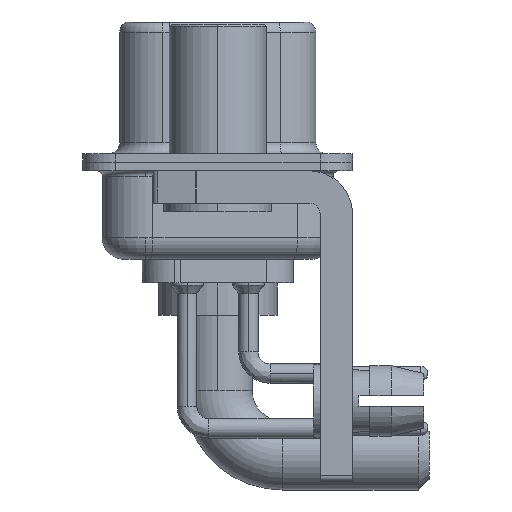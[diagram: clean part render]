
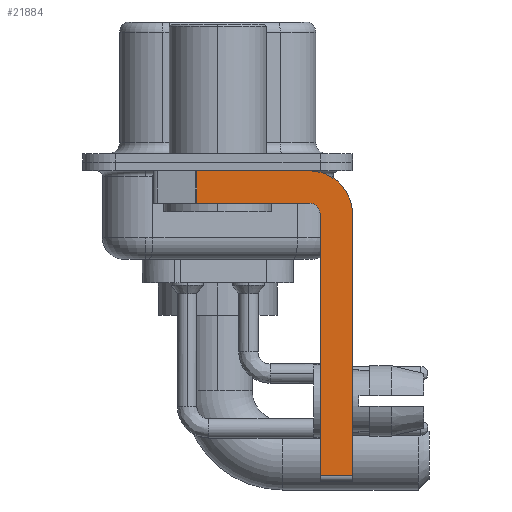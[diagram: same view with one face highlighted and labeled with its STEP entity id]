
A CAD part, left-side view. The second image highlights one B-rep face of the part: STEP entity #21884.
In plain terms, the highlighted planar face has unit normal (-1, 0, 0).
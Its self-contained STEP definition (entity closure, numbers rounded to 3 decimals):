
#239 = CARTESIAN_POINT ( 'NONE',  ( -2.9, 3., -0.4 ) ) ;
#353 = VERTEX_POINT ( 'NONE', #10017 ) ;
#521 = VERTEX_POINT ( 'NONE', #20869 ) ;
#617 = EDGE_CURVE ( 'NONE', #521, #15076, #24354, .T. ) ;
#702 = VECTOR ( 'NONE', #2770, 1000. ) ;
#852 = LINE ( 'NONE', #6659, #13976 ) ;
#1136 = DIRECTION ( 'NONE',  ( 0., 0., 1. ) ) ;
#1795 = DIRECTION ( 'NONE',  ( 0., 0., -1. ) ) ;
#1837 = EDGE_LOOP ( 'NONE', ( #18274, #26027, #17618, #20742, #22426, #16572, #10650, #2197 ) ) ;
#2197 = ORIENTED_EDGE ( 'NONE', *, *, #8988, .F. ) ;
#2770 = DIRECTION ( 'NONE',  ( 0., 1., 0. ) ) ;
#2832 = CARTESIAN_POINT ( 'NONE',  ( -2.9, -4.25, -0.4 ) ) ;
#2999 = DIRECTION ( 'NONE',  ( 0., -1., 0. ) ) ;
#4665 = LINE ( 'NONE', #6548, #12207 ) ;
#4983 = VERTEX_POINT ( 'NONE', #22659 ) ;
#5215 = DIRECTION ( 'NONE',  ( 0., 0., -1. ) ) ;
#5569 = AXIS2_PLACEMENT_3D ( 'NONE', #19363, #12936, #1136 ) ;
#5831 = VECTOR ( 'NONE', #2999, 1000. ) ;
#6110 = CARTESIAN_POINT ( 'NONE',  ( -2.9, -4.25, -2.4 ) ) ;
#6245 = PLANE ( 'NONE',  #14432 ) ;
#6363 = CARTESIAN_POINT ( 'NONE',  ( -2.9, -6.25, -14.55 ) ) ;
#6548 = CARTESIAN_POINT ( 'NONE',  ( -2.9, 0.978, -1.9 ) ) ;
#6659 = CARTESIAN_POINT ( 'NONE',  ( -2.9, -4.75, -14.8 ) ) ;
#6755 = EDGE_CURVE ( 'NONE', #17027, #9769, #16988, .T. ) ;
#8127 = CARTESIAN_POINT ( 'NONE',  ( -2.9, -4.25, -2.4 ) ) ;
#8738 = EDGE_CURVE ( 'NONE', #17027, #353, #4665, .T. ) ;
#8900 = VERTEX_POINT ( 'NONE', #23530 ) ;
#8988 = EDGE_CURVE ( 'NONE', #9769, #4983, #14767, .T. ) ;
#9285 = EDGE_CURVE ( 'NONE', #8900, #18835, #15437, .T. ) ;
#9769 = VERTEX_POINT ( 'NONE', #2832 ) ;
#10017 = CARTESIAN_POINT ( 'NONE',  ( -2.9, 0.978, -1.9 ) ) ;
#10063 = EDGE_CURVE ( 'NONE', #15076, #353, #10691, .T. ) ;
#10650 = ORIENTED_EDGE ( 'NONE', *, *, #15580, .F. ) ;
#10691 = LINE ( 'NONE', #23267, #702 ) ;
#10974 = CARTESIAN_POINT ( 'NONE',  ( -2.9, -6.25, -2.4 ) ) ;
#12207 = VECTOR ( 'NONE', #23264, 1000. ) ;
#12550 = VECTOR ( 'NONE', #14710, 1000. ) ;
#12936 = DIRECTION ( 'NONE',  ( -1., 0., 0. ) ) ;
#13976 = VECTOR ( 'NONE', #25398, 1000. ) ;
#14268 = DIRECTION ( 'NONE',  ( 0., 0., -1. ) ) ;
#14432 = AXIS2_PLACEMENT_3D ( 'NONE', #6110, #16512, #1795 ) ;
#14710 = DIRECTION ( 'NONE',  ( 0., -1., 0. ) ) ;
#14767 = CIRCLE ( 'NONE', #20353, 2. ) ;
#14912 = VECTOR ( 'NONE', #5215, 1000. ) ;
#15076 = VERTEX_POINT ( 'NONE', #17545 ) ;
#15437 = LINE ( 'NONE', #25775, #5831 ) ;
#15580 = EDGE_CURVE ( 'NONE', #4983, #18835, #19531, .T. ) ;
#16030 = CARTESIAN_POINT ( 'NONE',  ( -2.9, 0.978, -0.4 ) ) ;
#16512 = DIRECTION ( 'NONE',  ( 1., 0., 0. ) ) ;
#16572 = ORIENTED_EDGE ( 'NONE', *, *, #9285, .T. ) ;
#16988 = LINE ( 'NONE', #239, #12550 ) ;
#17027 = VERTEX_POINT ( 'NONE', #16030 ) ;
#17545 = CARTESIAN_POINT ( 'NONE',  ( -2.9, -4.25, -1.9 ) ) ;
#17618 = ORIENTED_EDGE ( 'NONE', *, *, #10063, .F. ) ;
#18274 = ORIENTED_EDGE ( 'NONE', *, *, #6755, .F. ) ;
#18835 = VERTEX_POINT ( 'NONE', #6363 ) ;
#19363 = CARTESIAN_POINT ( 'NONE',  ( -2.9, -4.25, -2.4 ) ) ;
#19531 = LINE ( 'NONE', #10974, #14912 ) ;
#19896 = DIRECTION ( 'NONE',  ( 1., 0., 0. ) ) ;
#20353 = AXIS2_PLACEMENT_3D ( 'NONE', #8127, #19896, #14268 ) ;
#20742 = ORIENTED_EDGE ( 'NONE', *, *, #617, .F. ) ;
#20869 = CARTESIAN_POINT ( 'NONE',  ( -2.9, -4.75, -2.4 ) ) ;
#21609 = EDGE_CURVE ( 'NONE', #8900, #521, #852, .T. ) ;
#21884 = ADVANCED_FACE ( 'NONE', ( #26183 ), #6245, .F. ) ;
#22426 = ORIENTED_EDGE ( 'NONE', *, *, #21609, .F. ) ;
#22659 = CARTESIAN_POINT ( 'NONE',  ( -2.9, -6.25, -2.4 ) ) ;
#23264 = DIRECTION ( 'NONE',  ( 0., 0., -1. ) ) ;
#23267 = CARTESIAN_POINT ( 'NONE',  ( -2.9, -4.25, -1.9 ) ) ;
#23530 = CARTESIAN_POINT ( 'NONE',  ( -2.9, -4.75, -14.55 ) ) ;
#24354 = CIRCLE ( 'NONE', #5569, 0.5 ) ;
#25398 = DIRECTION ( 'NONE',  ( 0., 0., 1. ) ) ;
#25775 = CARTESIAN_POINT ( 'NONE',  ( -2.9, -4.25, -14.55 ) ) ;
#26027 = ORIENTED_EDGE ( 'NONE', *, *, #8738, .T. ) ;
#26183 = FACE_OUTER_BOUND ( 'NONE', #1837, .T. ) ;
